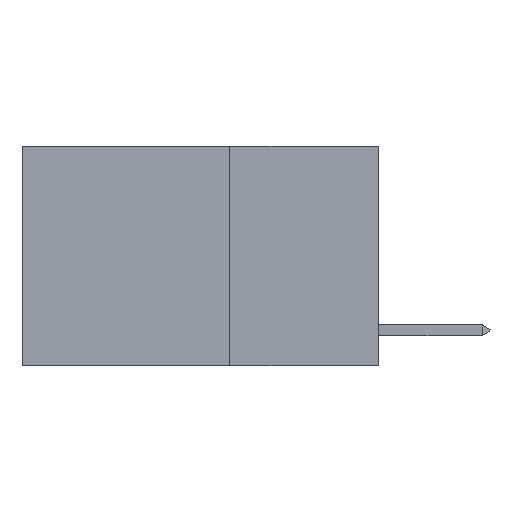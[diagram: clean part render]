
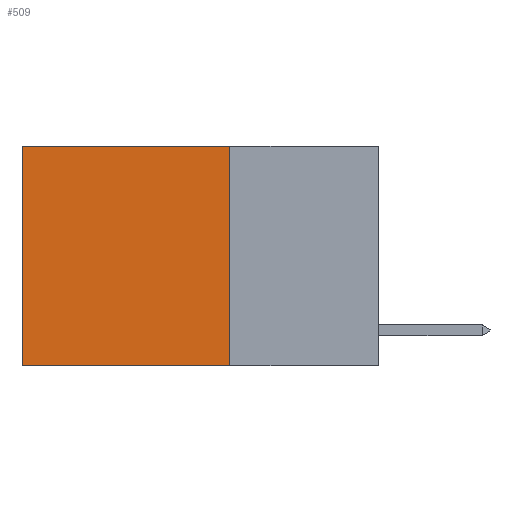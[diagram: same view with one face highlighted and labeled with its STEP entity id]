
A CAD part, left-side view. The second image highlights one B-rep face of the part: STEP entity #509.
In plain terms, the highlighted planar face has unit normal (-1, 0, 0).
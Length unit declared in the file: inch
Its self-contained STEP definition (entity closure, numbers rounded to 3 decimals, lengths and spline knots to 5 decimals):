
#509 = ADVANCED_FACE ( 'NONE', ( #19841 ), #19961, .F. ) ;
#1032 = ORIENTED_EDGE ( 'NONE', *, *, #14318, .T. ) ;
#1041 = VECTOR ( 'NONE', #8194, 39.37008 ) ;
#1455 = CARTESIAN_POINT ( 'NONE',  ( 0.2625, 0.6, 0. ) ) ;
#2689 = CARTESIAN_POINT ( 'NONE',  ( 0.2625, 0.25, -0.37 ) ) ;
#3163 = LINE ( 'NONE', #1455, #22274 ) ;
#3910 = LINE ( 'NONE', #8066, #1041 ) ;
#4305 = ORIENTED_EDGE ( 'NONE', *, *, #23303, .F. ) ;
#4416 = LINE ( 'NONE', #2689, #21056 ) ;
#5075 = LINE ( 'NONE', #7261, #21516 ) ;
#7261 = CARTESIAN_POINT ( 'NONE',  ( 0.2625, 0.25, 0. ) ) ;
#8066 = CARTESIAN_POINT ( 'NONE',  ( 0.2625, 0.25, 0. ) ) ;
#8194 = DIRECTION ( 'NONE',  ( 0., 1., 0. ) ) ;
#8259 = CARTESIAN_POINT ( 'NONE',  ( 0.2625, 0.6, -0.37 ) ) ;
#10181 = VERTEX_POINT ( 'NONE', #8259 ) ;
#10408 = CARTESIAN_POINT ( 'NONE',  ( 0.2625, 0.6, 0. ) ) ;
#11600 = DIRECTION ( 'NONE',  ( 0., 1., 0. ) ) ;
#11684 = VERTEX_POINT ( 'NONE', #13911 ) ;
#12480 = VERTEX_POINT ( 'NONE', #22102 ) ;
#12994 = AXIS2_PLACEMENT_3D ( 'NONE', #14054, #14295, #23740 ) ;
#13703 = ORIENTED_EDGE ( 'NONE', *, *, #15739, .F. ) ;
#13911 = CARTESIAN_POINT ( 'NONE',  ( 0.2625, 0.25, -0.37 ) ) ;
#14054 = CARTESIAN_POINT ( 'NONE',  ( 0.2625, 0.25, 0. ) ) ;
#14295 = DIRECTION ( 'NONE',  ( 1., 0., 0. ) ) ;
#14318 = EDGE_CURVE ( 'NONE', #12480, #16115, #3910, .T. ) ;
#14735 = DIRECTION ( 'NONE',  ( 0., 0., -1. ) ) ;
#15185 = EDGE_LOOP ( 'NONE', ( #18353, #13703, #4305, #1032 ) ) ;
#15739 = EDGE_CURVE ( 'NONE', #11684, #10181, #4416, .T. ) ;
#16115 = VERTEX_POINT ( 'NONE', #10408 ) ;
#18353 = ORIENTED_EDGE ( 'NONE', *, *, #23141, .T. ) ;
#19841 = FACE_OUTER_BOUND ( 'NONE', #15185, .T. ) ;
#19961 = PLANE ( 'NONE',  #12994 ) ;
#20448 = DIRECTION ( 'NONE',  ( 0., 0., -1. ) ) ;
#21056 = VECTOR ( 'NONE', #11600, 39.37008 ) ;
#21516 = VECTOR ( 'NONE', #14735, 39.37008 ) ;
#22102 = CARTESIAN_POINT ( 'NONE',  ( 0.2625, 0.25, 0. ) ) ;
#22274 = VECTOR ( 'NONE', #20448, 39.37008 ) ;
#23141 = EDGE_CURVE ( 'NONE', #16115, #10181, #3163, .T. ) ;
#23303 = EDGE_CURVE ( 'NONE', #12480, #11684, #5075, .T. ) ;
#23740 = DIRECTION ( 'NONE',  ( 0., 0., -1. ) ) ;
